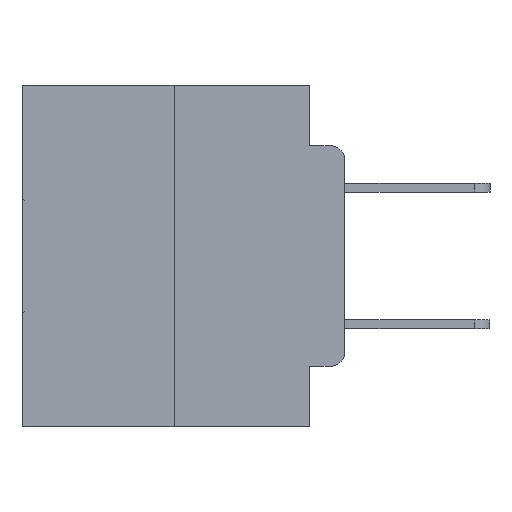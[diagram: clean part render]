
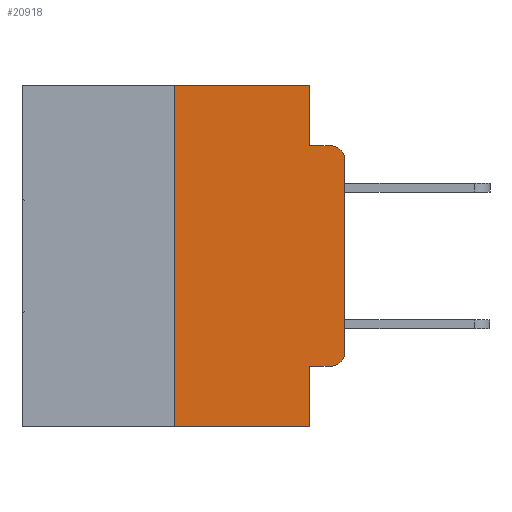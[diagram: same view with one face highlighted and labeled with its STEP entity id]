
A CAD part, left-side view. The second image highlights one B-rep face of the part: STEP entity #20918.
In plain terms, the highlighted planar face has unit normal (-1, 0, 0).
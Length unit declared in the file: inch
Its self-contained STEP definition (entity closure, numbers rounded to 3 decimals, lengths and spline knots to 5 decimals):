
#195 = VERTEX_POINT ( 'NONE', #6070 ) ;
#262 = CARTESIAN_POINT ( 'NONE',  ( 0., 0.051, 0. ) ) ;
#1119 = ORIENTED_EDGE ( 'NONE', *, *, #25277, .T. ) ;
#1351 = EDGE_CURVE ( 'NONE', #28360, #15829, #5425, .T. ) ;
#2255 = LINE ( 'NONE', #4418, #26217 ) ;
#2823 = DIRECTION ( 'NONE',  ( -1., 0., 0. ) ) ;
#2939 = DIRECTION ( 'NONE',  ( 0., 0., -1. ) ) ;
#3203 = CARTESIAN_POINT ( 'NONE',  ( 0., 0., 0. ) ) ;
#3760 = DIRECTION ( 'NONE',  ( 1., 0., 0. ) ) ;
#3785 = EDGE_CURVE ( 'NONE', #8348, #14951, #19488, .T. ) ;
#4114 = CARTESIAN_POINT ( 'NONE',  ( 0., 0.02, -0.0885 ) ) ;
#4418 = CARTESIAN_POINT ( 'NONE',  ( 0., 0.051, -0.0885 ) ) ;
#4785 = CARTESIAN_POINT ( 'NONE',  ( 0., 0.25, 0. ) ) ;
#5057 = CARTESIAN_POINT ( 'NONE',  ( 0., 0.25, 0. ) ) ;
#5108 = VERTEX_POINT ( 'NONE', #26001 ) ;
#5425 = LINE ( 'NONE', #3203, #17070 ) ;
#6044 = CARTESIAN_POINT ( 'NONE',  ( 0., 0.473, 0. ) ) ;
#6070 = CARTESIAN_POINT ( 'NONE',  ( 0., 0.02, -0.4115 ) ) ;
#6095 = AXIS2_PLACEMENT_3D ( 'NONE', #16828, #2823, #19134 ) ;
#6371 = ORIENTED_EDGE ( 'NONE', *, *, #14582, .F. ) ;
#6774 = CARTESIAN_POINT ( 'NONE',  ( 0., 0.051, -0.5 ) ) ;
#7169 = FACE_OUTER_BOUND ( 'NONE', #25558, .T. ) ;
#7200 = CARTESIAN_POINT ( 'NONE',  ( 0., 0.473, -0.5 ) ) ;
#7443 = ORIENTED_EDGE ( 'NONE', *, *, #1351, .T. ) ;
#8196 = VECTOR ( 'NONE', #8965, 39.37008 ) ;
#8241 = DIRECTION ( 'NONE',  ( 0., -1., 0. ) ) ;
#8348 = VERTEX_POINT ( 'NONE', #4785 ) ;
#8603 = VERTEX_POINT ( 'NONE', #27973 ) ;
#8914 = ORIENTED_EDGE ( 'NONE', *, *, #20677, .F. ) ;
#8965 = DIRECTION ( 'NONE',  ( 0., -1., 0. ) ) ;
#9007 = VERTEX_POINT ( 'NONE', #6774 ) ;
#9512 = VERTEX_POINT ( 'NONE', #4114 ) ;
#9657 = LINE ( 'NONE', #22776, #8196 ) ;
#9833 = CIRCLE ( 'NONE', #6095, 0.02 ) ;
#10633 = CARTESIAN_POINT ( 'NONE',  ( 0., 0.473, 0. ) ) ;
#10693 = DIRECTION ( 'NONE',  ( 0., 0., 1. ) ) ;
#10782 = LINE ( 'NONE', #5057, #21567 ) ;
#11452 = EDGE_CURVE ( 'NONE', #195, #28360, #24442, .T. ) ;
#11908 = DIRECTION ( 'NONE',  ( 0., -1., 0. ) ) ;
#12237 = CARTESIAN_POINT ( 'NONE',  ( 0., 0., -0.1085 ) ) ;
#12991 = EDGE_CURVE ( 'NONE', #5108, #195, #9657, .T. ) ;
#13047 = VECTOR ( 'NONE', #2939, 39.37008 ) ;
#13538 = DIRECTION ( 'NONE',  ( -1., 0., 0. ) ) ;
#14426 = CARTESIAN_POINT ( 'NONE',  ( 0., 0., -0.3915 ) ) ;
#14582 = EDGE_CURVE ( 'NONE', #5108, #9007, #26747, .T. ) ;
#14663 = CARTESIAN_POINT ( 'NONE',  ( 0., 0.051, 0. ) ) ;
#14951 = VERTEX_POINT ( 'NONE', #19933 ) ;
#15134 = ORIENTED_EDGE ( 'NONE', *, *, #3785, .F. ) ;
#15431 = PLANE ( 'NONE',  #27231 ) ;
#15829 = VERTEX_POINT ( 'NONE', #12237 ) ;
#16454 = VECTOR ( 'NONE', #11908, 39.37008 ) ;
#16671 = DIRECTION ( 'NONE',  ( 0., 0., 1. ) ) ;
#16828 = CARTESIAN_POINT ( 'NONE',  ( 0., 0.02, -0.1085 ) ) ;
#17070 = VECTOR ( 'NONE', #10693, 39.37008 ) ;
#17181 = LINE ( 'NONE', #7200, #16454 ) ;
#17645 = EDGE_CURVE ( 'NONE', #23887, #8348, #10782, .T. ) ;
#18753 = LINE ( 'NONE', #14663, #13047 ) ;
#19134 = DIRECTION ( 'NONE',  ( 0., 0., -1. ) ) ;
#19488 = LINE ( 'NONE', #10633, #21235 ) ;
#19566 = EDGE_CURVE ( 'NONE', #23887, #9007, #17181, .T. ) ;
#19775 = ORIENTED_EDGE ( 'NONE', *, *, #22212, .F. ) ;
#19933 = CARTESIAN_POINT ( 'NONE',  ( 0., 0.051, 0. ) ) ;
#19948 = VECTOR ( 'NONE', #25890, 39.37008 ) ;
#20021 = DIRECTION ( 'NONE',  ( 0., 0., -1. ) ) ;
#20100 = AXIS2_PLACEMENT_3D ( 'NONE', #27252, #13538, #29497 ) ;
#20131 = ORIENTED_EDGE ( 'NONE', *, *, #11452, .T. ) ;
#20641 = DIRECTION ( 'NONE',  ( 0., -1., 0. ) ) ;
#20677 = EDGE_CURVE ( 'NONE', #14951, #8603, #18753, .T. ) ;
#20918 = ADVANCED_FACE ( 'NONE', ( #7169 ), #15431, .F. ) ;
#21185 = ORIENTED_EDGE ( 'NONE', *, *, #17645, .F. ) ;
#21235 = VECTOR ( 'NONE', #8241, 39.37008 ) ;
#21567 = VECTOR ( 'NONE', #16671, 39.37008 ) ;
#22212 = EDGE_CURVE ( 'NONE', #8603, #9512, #2255, .T. ) ;
#22617 = ORIENTED_EDGE ( 'NONE', *, *, #19566, .T. ) ;
#22776 = CARTESIAN_POINT ( 'NONE',  ( 0., 0.051, -0.4115 ) ) ;
#23887 = VERTEX_POINT ( 'NONE', #25391 ) ;
#24442 = CIRCLE ( 'NONE', #20100, 0.02 ) ;
#25277 = EDGE_CURVE ( 'NONE', #15829, #9512, #9833, .T. ) ;
#25391 = CARTESIAN_POINT ( 'NONE',  ( 0., 0.25, -0.5 ) ) ;
#25558 = EDGE_LOOP ( 'NONE', ( #7443, #1119, #19775, #8914, #15134, #21185, #22617, #6371, #26223, #20131 ) ) ;
#25890 = DIRECTION ( 'NONE',  ( 0., 0., -1. ) ) ;
#26001 = CARTESIAN_POINT ( 'NONE',  ( 0., 0.051, -0.4115 ) ) ;
#26217 = VECTOR ( 'NONE', #20641, 39.37008 ) ;
#26223 = ORIENTED_EDGE ( 'NONE', *, *, #12991, .T. ) ;
#26747 = LINE ( 'NONE', #262, #19948 ) ;
#27231 = AXIS2_PLACEMENT_3D ( 'NONE', #6044, #3760, #20021 ) ;
#27252 = CARTESIAN_POINT ( 'NONE',  ( 0., 0.02, -0.3915 ) ) ;
#27973 = CARTESIAN_POINT ( 'NONE',  ( 0., 0.051, -0.0885 ) ) ;
#28360 = VERTEX_POINT ( 'NONE', #14426 ) ;
#29497 = DIRECTION ( 'NONE',  ( 0., 0., -1. ) ) ;
